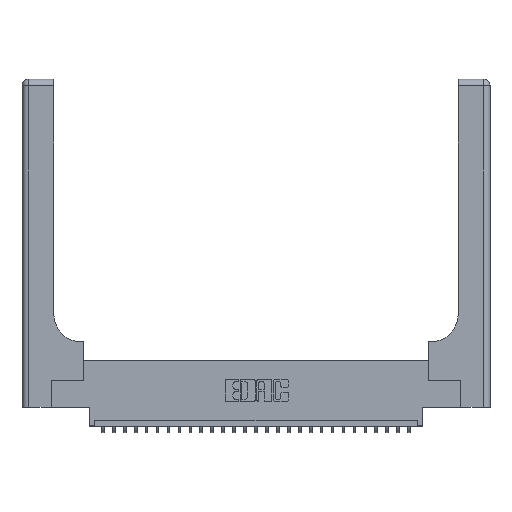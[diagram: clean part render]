
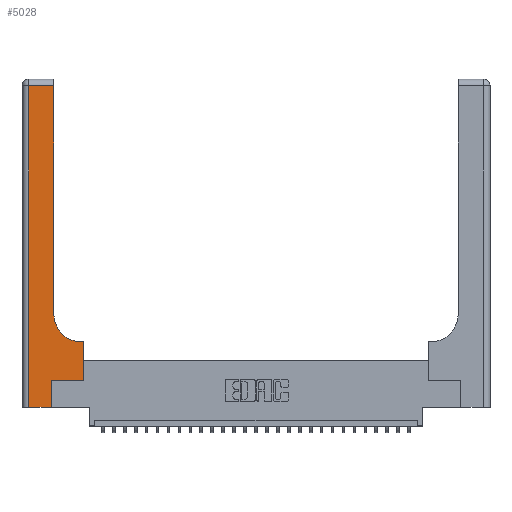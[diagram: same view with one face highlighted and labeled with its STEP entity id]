
A CAD part, top view. The second image highlights one B-rep face of the part: STEP entity #5028.
In plain terms, the highlighted planar face has unit normal (0, 0, 1).
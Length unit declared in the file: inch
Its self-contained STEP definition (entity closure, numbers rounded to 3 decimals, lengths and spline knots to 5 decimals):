
#148 = LINE ( 'NONE', #14859, #2974 ) ;
#274 = DIRECTION ( 'NONE',  ( 0., 1., 0. ) ) ;
#359 = CARTESIAN_POINT ( 'NONE',  ( 0.5585, 0.25, 0.37 ) ) ;
#1087 = EDGE_CURVE ( 'NONE', #23787, #8145, #27060, .T. ) ;
#1421 = DIRECTION ( 'NONE',  ( 0., -1., 0. ) ) ;
#2225 = VECTOR ( 'NONE', #7508, 39.37008 ) ;
#2244 = LINE ( 'NONE', #9206, #11387 ) ;
#2245 = CARTESIAN_POINT ( 'NONE',  ( 0.269, 0., 0.37 ) ) ;
#2480 = LINE ( 'NONE', #13487, #10958 ) ;
#2942 = AXIS2_PLACEMENT_3D ( 'NONE', #17910, #4574, #22648 ) ;
#2974 = VECTOR ( 'NONE', #1421, 39.37008 ) ;
#3256 = EDGE_CURVE ( 'NONE', #26617, #17332, #9764, .T. ) ;
#3364 = AXIS2_PLACEMENT_3D ( 'NONE', #8201, #23908, #26145 ) ;
#3791 = CARTESIAN_POINT ( 'NONE',  ( 0.2915, 0.85, 0.37 ) ) ;
#3903 = ORIENTED_EDGE ( 'NONE', *, *, #7190, .T. ) ;
#4112 = VECTOR ( 'NONE', #24968, 39.37008 ) ;
#4574 = DIRECTION ( 'NONE',  ( 0., 0., -1. ) ) ;
#5028 = ADVANCED_FACE ( 'NONE', ( #28875 ), #21676, .F. ) ;
#5733 = ORIENTED_EDGE ( 'NONE', *, *, #3256, .T. ) ;
#6314 = CARTESIAN_POINT ( 'NONE',  ( 0.5585, 0.6, 0.37 ) ) ;
#6424 = EDGE_CURVE ( 'NONE', #8145, #13714, #2244, .T. ) ;
#7190 = EDGE_CURVE ( 'NONE', #19771, #18735, #148, .T. ) ;
#7508 = DIRECTION ( 'NONE',  ( -1., 0., 0. ) ) ;
#8075 = ORIENTED_EDGE ( 'NONE', *, *, #1087, .T. ) ;
#8145 = VERTEX_POINT ( 'NONE', #3791 ) ;
#8201 = CARTESIAN_POINT ( 'NONE',  ( 0., 3., 0.37 ) ) ;
#9046 = VECTOR ( 'NONE', #26644, 39.37008 ) ;
#9206 = CARTESIAN_POINT ( 'NONE',  ( 0.2915, 3., 0.37 ) ) ;
#9764 = LINE ( 'NONE', #2245, #9046 ) ;
#9958 = EDGE_CURVE ( 'NONE', #19551, #23787, #20132, .T. ) ;
#10431 = CARTESIAN_POINT ( 'NONE',  ( 0.2915, 2.94, 0.37 ) ) ;
#10958 = VECTOR ( 'NONE', #24829, 39.37008 ) ;
#11121 = LINE ( 'NONE', #27136, #27184 ) ;
#11138 = ORIENTED_EDGE ( 'NONE', *, *, #24530, .T. ) ;
#11387 = VECTOR ( 'NONE', #274, 39.37008 ) ;
#11478 = CARTESIAN_POINT ( 'NONE',  ( 0., 0., 0.37 ) ) ;
#13287 = EDGE_CURVE ( 'NONE', #18735, #26617, #17772, .T. ) ;
#13487 = CARTESIAN_POINT ( 'NONE',  ( 0.5585, 0.25, 0.37 ) ) ;
#13714 = VERTEX_POINT ( 'NONE', #10431 ) ;
#13835 = ORIENTED_EDGE ( 'NONE', *, *, #17450, .T. ) ;
#14385 = EDGE_CURVE ( 'NONE', #13714, #19771, #11121, .T. ) ;
#14859 = CARTESIAN_POINT ( 'NONE',  ( 0.06, 3., 0.37 ) ) ;
#15131 = VERTEX_POINT ( 'NONE', #359 ) ;
#16007 = DIRECTION ( 'NONE',  ( 1., 0., 0. ) ) ;
#16718 = CARTESIAN_POINT ( 'NONE',  ( 0.06, 0., 0.37 ) ) ;
#17332 = VERTEX_POINT ( 'NONE', #25798 ) ;
#17450 = EDGE_CURVE ( 'NONE', #17332, #15131, #18296, .T. ) ;
#17772 = LINE ( 'NONE', #11478, #4112 ) ;
#17886 = ORIENTED_EDGE ( 'NONE', *, *, #9958, .T. ) ;
#17910 = CARTESIAN_POINT ( 'NONE',  ( 0.5415, 0.85, 0.37 ) ) ;
#18296 = LINE ( 'NONE', #24912, #27393 ) ;
#18486 = CARTESIAN_POINT ( 'NONE',  ( 0.06, 2.94, 0.37 ) ) ;
#18735 = VERTEX_POINT ( 'NONE', #16718 ) ;
#19551 = VERTEX_POINT ( 'NONE', #6314 ) ;
#19771 = VERTEX_POINT ( 'NONE', #18486 ) ;
#20132 = LINE ( 'NONE', #27501, #2225 ) ;
#20405 = ORIENTED_EDGE ( 'NONE', *, *, #14385, .T. ) ;
#21676 = PLANE ( 'NONE',  #3364 ) ;
#21747 = EDGE_LOOP ( 'NONE', ( #23363, #20405, #3903, #25391, #5733, #13835, #11138, #17886, #8075 ) ) ;
#21857 = CARTESIAN_POINT ( 'NONE',  ( 0.5415, 0.6, 0.37 ) ) ;
#22648 = DIRECTION ( 'NONE',  ( 1., 0., 0. ) ) ;
#23363 = ORIENTED_EDGE ( 'NONE', *, *, #6424, .T. ) ;
#23787 = VERTEX_POINT ( 'NONE', #21857 ) ;
#23908 = DIRECTION ( 'NONE',  ( 0., 0., -1. ) ) ;
#24530 = EDGE_CURVE ( 'NONE', #15131, #19551, #2480, .T. ) ;
#24643 = DIRECTION ( 'NONE',  ( -1., 0., 0. ) ) ;
#24829 = DIRECTION ( 'NONE',  ( 0., 1., 0. ) ) ;
#24912 = CARTESIAN_POINT ( 'NONE',  ( 0.269, 0.25, 0.37 ) ) ;
#24968 = DIRECTION ( 'NONE',  ( 1., 0., 0. ) ) ;
#25391 = ORIENTED_EDGE ( 'NONE', *, *, #13287, .T. ) ;
#25798 = CARTESIAN_POINT ( 'NONE',  ( 0.269, 0.25, 0.37 ) ) ;
#26145 = DIRECTION ( 'NONE',  ( -1., 0., 0. ) ) ;
#26458 = CARTESIAN_POINT ( 'NONE',  ( 0.269, 0., 0.37 ) ) ;
#26617 = VERTEX_POINT ( 'NONE', #26458 ) ;
#26644 = DIRECTION ( 'NONE',  ( 0., 1., 0. ) ) ;
#27060 = CIRCLE ( 'NONE', #2942, 0.25 ) ;
#27136 = CARTESIAN_POINT ( 'NONE',  ( 0., 2.94, 0.37 ) ) ;
#27184 = VECTOR ( 'NONE', #24643, 39.37008 ) ;
#27393 = VECTOR ( 'NONE', #16007, 39.37008 ) ;
#27501 = CARTESIAN_POINT ( 'NONE',  ( 0.2915, 0.6, 0.37 ) ) ;
#28875 = FACE_OUTER_BOUND ( 'NONE', #21747, .T. ) ;
